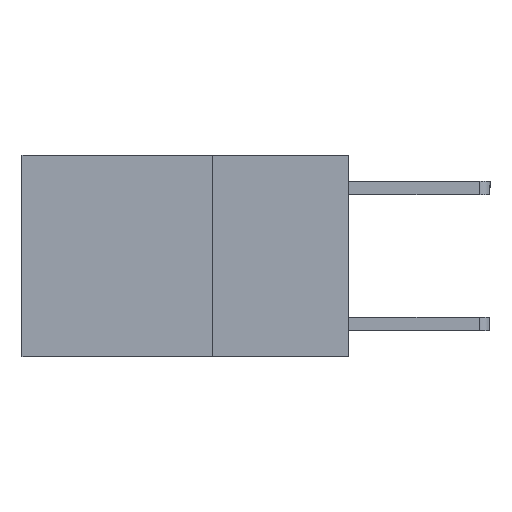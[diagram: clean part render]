
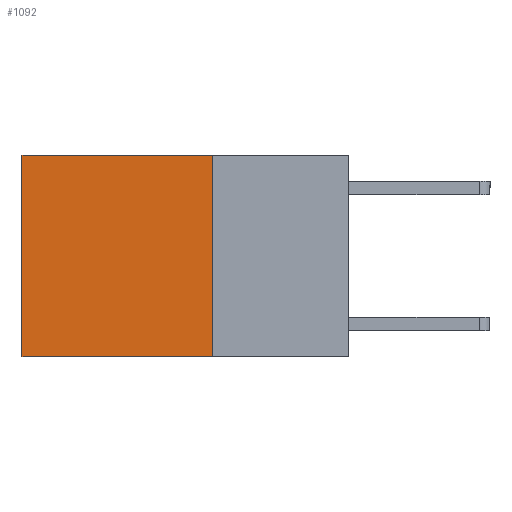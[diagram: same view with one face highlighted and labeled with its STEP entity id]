
A CAD part, left-side view. The second image highlights one B-rep face of the part: STEP entity #1092.
In plain terms, the highlighted planar face has unit normal (-1, 0, 0).
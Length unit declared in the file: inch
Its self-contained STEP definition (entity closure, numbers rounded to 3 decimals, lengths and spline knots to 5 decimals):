
#195 = CARTESIAN_POINT ( 'NONE',  ( 0.2625, 0.25, -0.37 ) ) ;
#478 = VERTEX_POINT ( 'NONE', #2875 ) ;
#580 = AXIS2_PLACEMENT_3D ( 'NONE', #7837, #767, #2326 ) ;
#610 = CARTESIAN_POINT ( 'NONE',  ( 0.2625, 0.6, 0. ) ) ;
#677 = CARTESIAN_POINT ( 'NONE',  ( 0.2625, 0.6, 0. ) ) ;
#767 = DIRECTION ( 'NONE',  ( 1., 0., 0. ) ) ;
#814 = LINE ( 'NONE', #4711, #2792 ) ;
#972 = CARTESIAN_POINT ( 'NONE',  ( 0.2625, 0.6, -0.37 ) ) ;
#1092 = ADVANCED_FACE ( 'NONE', ( #6177 ), #10172, .F. ) ;
#1325 = CARTESIAN_POINT ( 'NONE',  ( 0.2625, 0.25, 0. ) ) ;
#1428 = ORIENTED_EDGE ( 'NONE', *, *, #2342, .F. ) ;
#1833 = EDGE_LOOP ( 'NONE', ( #8027, #7300, #1428, #10249 ) ) ;
#2095 = DIRECTION ( 'NONE',  ( 0., 0., -1. ) ) ;
#2326 = DIRECTION ( 'NONE',  ( 0., 0., -1. ) ) ;
#2342 = EDGE_CURVE ( 'NONE', #478, #3076, #814, .T. ) ;
#2789 = VECTOR ( 'NONE', #4485, 39.37008 ) ;
#2792 = VECTOR ( 'NONE', #9449, 39.37008 ) ;
#2875 = CARTESIAN_POINT ( 'NONE',  ( 0.2625, 0.25, 0. ) ) ;
#3076 = VERTEX_POINT ( 'NONE', #10198 ) ;
#3816 = LINE ( 'NONE', #1325, #2789 ) ;
#4374 = EDGE_CURVE ( 'NONE', #3076, #8570, #5014, .T. ) ;
#4485 = DIRECTION ( 'NONE',  ( 0., 1., 0. ) ) ;
#4573 = LINE ( 'NONE', #677, #7844 ) ;
#4711 = CARTESIAN_POINT ( 'NONE',  ( 0.2625, 0.25, 0. ) ) ;
#4770 = VECTOR ( 'NONE', #4912, 39.37008 ) ;
#4912 = DIRECTION ( 'NONE',  ( 0., 1., 0. ) ) ;
#5014 = LINE ( 'NONE', #195, #4770 ) ;
#6081 = VERTEX_POINT ( 'NONE', #610 ) ;
#6177 = FACE_OUTER_BOUND ( 'NONE', #1833, .T. ) ;
#7300 = ORIENTED_EDGE ( 'NONE', *, *, #4374, .F. ) ;
#7695 = EDGE_CURVE ( 'NONE', #478, #6081, #3816, .T. ) ;
#7837 = CARTESIAN_POINT ( 'NONE',  ( 0.2625, 0.25, 0. ) ) ;
#7844 = VECTOR ( 'NONE', #2095, 39.37008 ) ;
#8027 = ORIENTED_EDGE ( 'NONE', *, *, #9834, .T. ) ;
#8570 = VERTEX_POINT ( 'NONE', #972 ) ;
#9449 = DIRECTION ( 'NONE',  ( 0., 0., -1. ) ) ;
#9834 = EDGE_CURVE ( 'NONE', #6081, #8570, #4573, .T. ) ;
#10172 = PLANE ( 'NONE',  #580 ) ;
#10198 = CARTESIAN_POINT ( 'NONE',  ( 0.2625, 0.25, -0.37 ) ) ;
#10249 = ORIENTED_EDGE ( 'NONE', *, *, #7695, .T. ) ;
